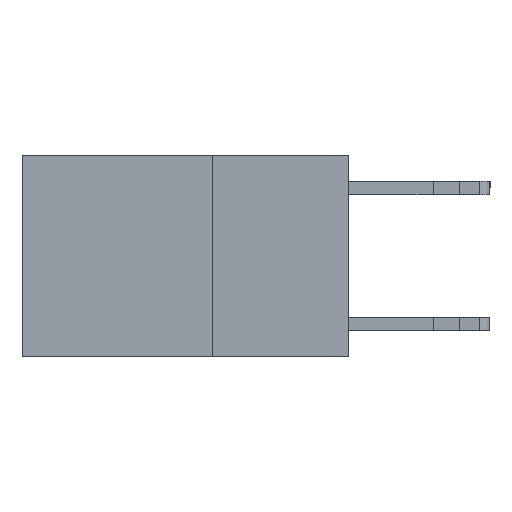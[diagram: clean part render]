
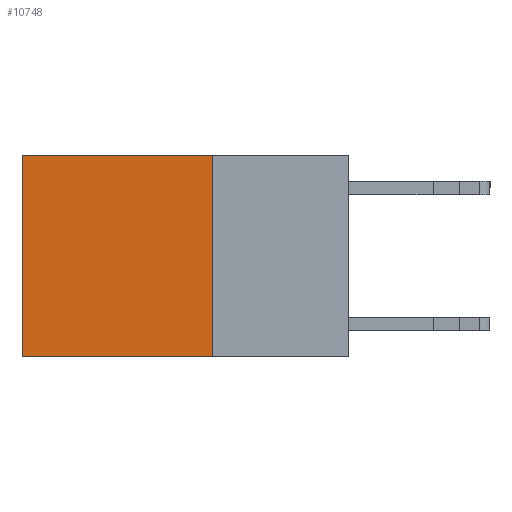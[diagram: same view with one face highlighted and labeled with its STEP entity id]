
A CAD part, left-side view. The second image highlights one B-rep face of the part: STEP entity #10748.
In plain terms, the highlighted planar face has unit normal (-1, 0, 0).
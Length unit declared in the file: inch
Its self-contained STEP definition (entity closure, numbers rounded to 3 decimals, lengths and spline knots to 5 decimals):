
#590 = DIRECTION ( 'NONE',  ( 0., 0., -1. ) ) ;
#2413 = VECTOR ( 'NONE', #10249, 39.37008 ) ;
#2645 = FACE_OUTER_BOUND ( 'NONE', #17183, .T. ) ;
#2743 = LINE ( 'NONE', #4701, #2413 ) ;
#3133 = LINE ( 'NONE', #13238, #4953 ) ;
#4030 = DIRECTION ( 'NONE',  ( 1., 0., 0. ) ) ;
#4321 = PLANE ( 'NONE',  #13247 ) ;
#4482 = VERTEX_POINT ( 'NONE', #10179 ) ;
#4567 = EDGE_CURVE ( 'NONE', #4482, #7639, #2743, .T. ) ;
#4701 = CARTESIAN_POINT ( 'NONE',  ( 0.2625, 0.6, 0. ) ) ;
#4953 = VECTOR ( 'NONE', #590, 39.37008 ) ;
#5121 = CARTESIAN_POINT ( 'NONE',  ( 0.2625, 0.25, 0. ) ) ;
#5537 = VECTOR ( 'NONE', #7469, 39.37008 ) ;
#5637 = ORIENTED_EDGE ( 'NONE', *, *, #4567, .T. ) ;
#5926 = EDGE_CURVE ( 'NONE', #16502, #10844, #3133, .T. ) ;
#5984 = CARTESIAN_POINT ( 'NONE',  ( 0.2625, 0.25, -0.37 ) ) ;
#6120 = ORIENTED_EDGE ( 'NONE', *, *, #10792, .T. ) ;
#6611 = CARTESIAN_POINT ( 'NONE',  ( 0.2625, 0.6, -0.37 ) ) ;
#6988 = CARTESIAN_POINT ( 'NONE',  ( 0.2625, 0.25, 0. ) ) ;
#7469 = DIRECTION ( 'NONE',  ( 0., 1., 0. ) ) ;
#7639 = VERTEX_POINT ( 'NONE', #6611 ) ;
#8526 = VECTOR ( 'NONE', #8665, 39.37008 ) ;
#8665 = DIRECTION ( 'NONE',  ( 0., 1., 0. ) ) ;
#9782 = LINE ( 'NONE', #14018, #5537 ) ;
#10179 = CARTESIAN_POINT ( 'NONE',  ( 0.2625, 0.6, 0. ) ) ;
#10249 = DIRECTION ( 'NONE',  ( 0., 0., -1. ) ) ;
#10665 = CARTESIAN_POINT ( 'NONE',  ( 0.2625, 0.25, -0.37 ) ) ;
#10748 = ADVANCED_FACE ( 'NONE', ( #2645 ), #4321, .F. ) ;
#10792 = EDGE_CURVE ( 'NONE', #16502, #4482, #9782, .T. ) ;
#10844 = VERTEX_POINT ( 'NONE', #10665 ) ;
#12582 = LINE ( 'NONE', #5984, #8526 ) ;
#12854 = DIRECTION ( 'NONE',  ( 0., 0., -1. ) ) ;
#13238 = CARTESIAN_POINT ( 'NONE',  ( 0.2625, 0.25, 0. ) ) ;
#13247 = AXIS2_PLACEMENT_3D ( 'NONE', #6988, #4030, #12854 ) ;
#14018 = CARTESIAN_POINT ( 'NONE',  ( 0.2625, 0.25, 0. ) ) ;
#14506 = ORIENTED_EDGE ( 'NONE', *, *, #5926, .F. ) ;
#15410 = ORIENTED_EDGE ( 'NONE', *, *, #16074, .F. ) ;
#16074 = EDGE_CURVE ( 'NONE', #10844, #7639, #12582, .T. ) ;
#16502 = VERTEX_POINT ( 'NONE', #5121 ) ;
#17183 = EDGE_LOOP ( 'NONE', ( #5637, #15410, #14506, #6120 ) ) ;
